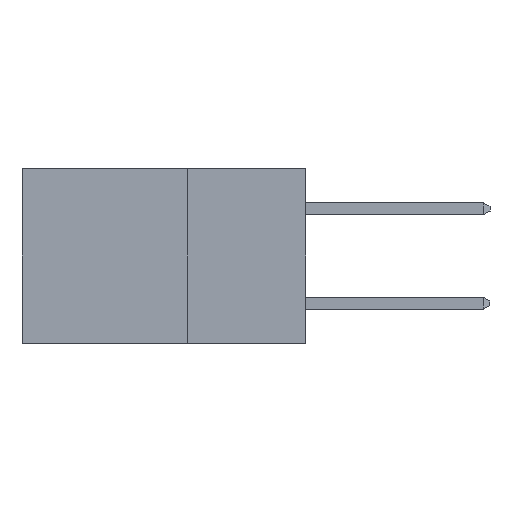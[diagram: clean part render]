
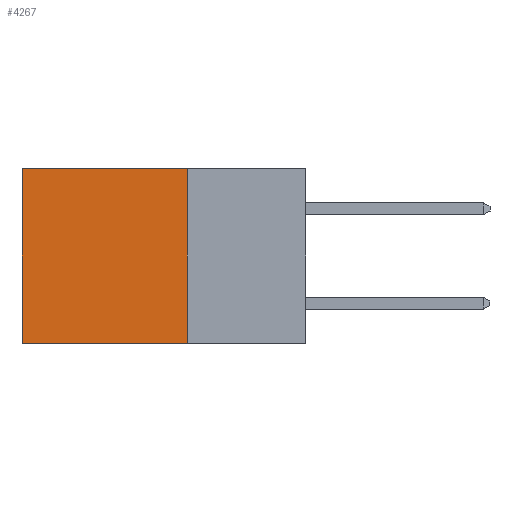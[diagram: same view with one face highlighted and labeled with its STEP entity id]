
A CAD part, left-side view. The second image highlights one B-rep face of the part: STEP entity #4267.
In plain terms, the highlighted planar face has unit normal (-1, 0, 0).
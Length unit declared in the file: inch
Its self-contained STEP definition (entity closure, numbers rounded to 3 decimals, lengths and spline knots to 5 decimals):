
#342 = EDGE_CURVE ( 'NONE', #1075, #1105, #3281, .T. ) ;
#665 = VECTOR ( 'NONE', #4057, 39.37008 ) ;
#1075 = VERTEX_POINT ( 'NONE', #6247 ) ;
#1105 = VERTEX_POINT ( 'NONE', #5753 ) ;
#1199 = AXIS2_PLACEMENT_3D ( 'NONE', #4319, #4273, #4842 ) ;
#1567 = ORIENTED_EDGE ( 'NONE', *, *, #7566, .T. ) ;
#1620 = VECTOR ( 'NONE', #1661, 39.37008 ) ;
#1661 = DIRECTION ( 'NONE',  ( 0., 1., 0. ) ) ;
#2237 = EDGE_LOOP ( 'NONE', ( #3286, #9478, #5622, #1567 ) ) ;
#2877 = LINE ( 'NONE', #5603, #6757 ) ;
#3149 = VERTEX_POINT ( 'NONE', #7015 ) ;
#3162 = VERTEX_POINT ( 'NONE', #7037 ) ;
#3281 = LINE ( 'NONE', #4187, #665 ) ;
#3286 = ORIENTED_EDGE ( 'NONE', *, *, #8549, .T. ) ;
#4057 = DIRECTION ( 'NONE',  ( 0., 0., -1. ) ) ;
#4187 = CARTESIAN_POINT ( 'NONE',  ( 0.298, 0.25, 0. ) ) ;
#4267 = ADVANCED_FACE ( 'NONE', ( #8667 ), #5216, .F. ) ;
#4273 = DIRECTION ( 'NONE',  ( 1., 0., 0. ) ) ;
#4319 = CARTESIAN_POINT ( 'NONE',  ( 0.298, 0.25, 0. ) ) ;
#4607 = LINE ( 'NONE', #5373, #7979 ) ;
#4837 = DIRECTION ( 'NONE',  ( 0., 1., 0. ) ) ;
#4842 = DIRECTION ( 'NONE',  ( 0., 0., -1. ) ) ;
#5216 = PLANE ( 'NONE',  #1199 ) ;
#5373 = CARTESIAN_POINT ( 'NONE',  ( 0.298, 0.6, 0. ) ) ;
#5603 = CARTESIAN_POINT ( 'NONE',  ( 0.298, 0.25, 0. ) ) ;
#5622 = ORIENTED_EDGE ( 'NONE', *, *, #342, .F. ) ;
#5682 = CARTESIAN_POINT ( 'NONE',  ( 0.298, 0.25, -0.37 ) ) ;
#5753 = CARTESIAN_POINT ( 'NONE',  ( 0.298, 0.25, -0.37 ) ) ;
#6247 = CARTESIAN_POINT ( 'NONE',  ( 0.298, 0.25, 0. ) ) ;
#6757 = VECTOR ( 'NONE', #4837, 39.37008 ) ;
#7015 = CARTESIAN_POINT ( 'NONE',  ( 0.298, 0.6, -0.37 ) ) ;
#7037 = CARTESIAN_POINT ( 'NONE',  ( 0.298, 0.6, 0. ) ) ;
#7566 = EDGE_CURVE ( 'NONE', #1075, #3162, #2877, .T. ) ;
#7979 = VECTOR ( 'NONE', #9201, 39.37008 ) ;
#8549 = EDGE_CURVE ( 'NONE', #3162, #3149, #4607, .T. ) ;
#8667 = FACE_OUTER_BOUND ( 'NONE', #2237, .T. ) ;
#9201 = DIRECTION ( 'NONE',  ( 0., 0., -1. ) ) ;
#9478 = ORIENTED_EDGE ( 'NONE', *, *, #10506, .F. ) ;
#10033 = LINE ( 'NONE', #5682, #1620 ) ;
#10506 = EDGE_CURVE ( 'NONE', #1105, #3149, #10033, .T. ) ;
